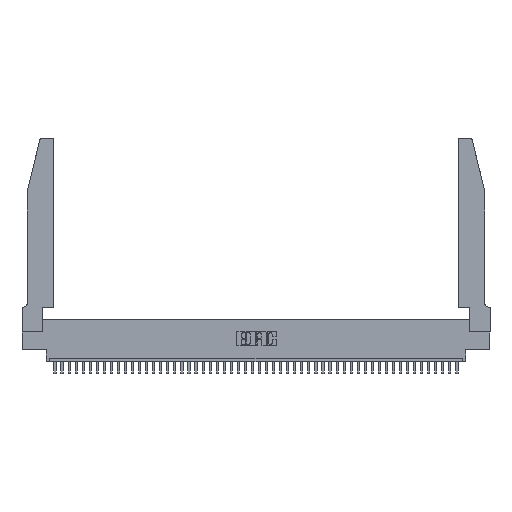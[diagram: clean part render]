
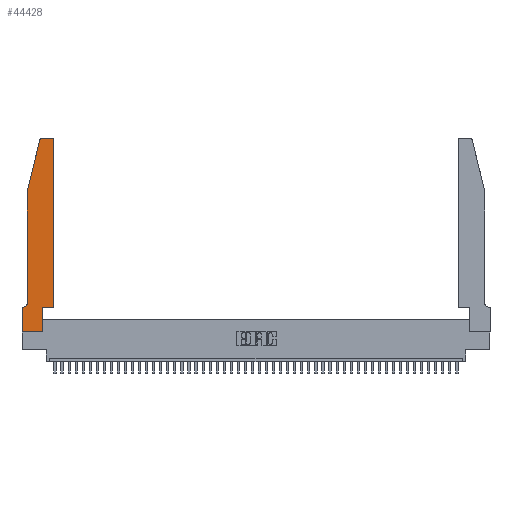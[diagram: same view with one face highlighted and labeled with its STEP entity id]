
A CAD part, top view. The second image highlights one B-rep face of the part: STEP entity #44428.
In plain terms, the highlighted planar face has unit normal (0, 0, 1).
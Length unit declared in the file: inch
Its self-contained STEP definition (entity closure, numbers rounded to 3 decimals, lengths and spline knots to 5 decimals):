
#929 = DIRECTION ( 'NONE',  ( -1., 0., 0. ) ) ;
#1763 = EDGE_CURVE ( 'NONE', #12668, #45169, #44004, .T. ) ;
#1873 = LINE ( 'NONE', #11984, #23789 ) ;
#2221 = EDGE_CURVE ( 'NONE', #45169, #33366, #1873, .T. ) ;
#2906 = EDGE_CURVE ( 'NONE', #33366, #6552, #17636, .T. ) ;
#4035 = ORIENTED_EDGE ( 'NONE', *, *, #28846, .T. ) ;
#4823 = VECTOR ( 'NONE', #13705, 39.37008 ) ;
#5790 = DIRECTION ( 'NONE',  ( 1., 0., 0. ) ) ;
#5920 = VERTEX_POINT ( 'NONE', #32987 ) ;
#6147 = EDGE_LOOP ( 'NONE', ( #6750, #25778, #36828, #45450, #25451, #10284, #23994, #35107, #44452, #25367, #8955, #4035 ) ) ;
#6552 = VERTEX_POINT ( 'NONE', #12943 ) ;
#6570 = EDGE_CURVE ( 'NONE', #5920, #10845, #46477, .T. ) ;
#6750 = ORIENTED_EDGE ( 'NONE', *, *, #9562, .T. ) ;
#7239 = CARTESIAN_POINT ( 'NONE',  ( 0.2865, 0.35, 0.37 ) ) ;
#8721 = LINE ( 'NONE', #35166, #18731 ) ;
#8955 = ORIENTED_EDGE ( 'NONE', *, *, #12081, .T. ) ;
#8992 = DIRECTION ( 'NONE',  ( -0.239, -0.971, 0. ) ) ;
#9445 = VERTEX_POINT ( 'NONE', #15338 ) ;
#9562 = EDGE_CURVE ( 'NONE', #10514, #5920, #22978, .T. ) ;
#10023 = EDGE_CURVE ( 'NONE', #6552, #16545, #29719, .T. ) ;
#10284 = ORIENTED_EDGE ( 'NONE', *, *, #2221, .T. ) ;
#10514 = VERTEX_POINT ( 'NONE', #44878 ) ;
#10845 = VERTEX_POINT ( 'NONE', #13922 ) ;
#11984 = CARTESIAN_POINT ( 'NONE',  ( 0.0755, 0.35, 0.37 ) ) ;
#12081 = EDGE_CURVE ( 'NONE', #36605, #31818, #8721, .T. ) ;
#12510 = FACE_OUTER_BOUND ( 'NONE', #6147, .T. ) ;
#12601 = VECTOR ( 'NONE', #39973, 39.37008 ) ;
#12668 = VERTEX_POINT ( 'NONE', #17203 ) ;
#12858 = PLANE ( 'NONE',  #36894 ) ;
#12943 = CARTESIAN_POINT ( 'NONE',  ( 0., 0., 0.37 ) ) ;
#13392 = CARTESIAN_POINT ( 'NONE',  ( 0.4505, 0.35, 0.37 ) ) ;
#13705 = DIRECTION ( 'NONE',  ( 1., 0., 0. ) ) ;
#13922 = CARTESIAN_POINT ( 'NONE',  ( 0.25487, 2.72718, 0.37 ) ) ;
#14198 = CARTESIAN_POINT ( 'NONE',  ( 0.0055, 0.35, 0.37 ) ) ;
#14454 = CARTESIAN_POINT ( 'NONE',  ( 0., 0.35, 0.37 ) ) ;
#15338 = CARTESIAN_POINT ( 'NONE',  ( 0.0755, 2., 0.37 ) ) ;
#15631 = VECTOR ( 'NONE', #17059, 39.37008 ) ;
#16433 = CARTESIAN_POINT ( 'NONE',  ( 0., 0.35, 0.37 ) ) ;
#16516 = CARTESIAN_POINT ( 'NONE',  ( 0.284, 2.72, 0.37 ) ) ;
#16545 = VERTEX_POINT ( 'NONE', #18893 ) ;
#17059 = DIRECTION ( 'NONE',  ( 1., 0., 0. ) ) ;
#17203 = CARTESIAN_POINT ( 'NONE',  ( 0.0755, 0.42, 0.37 ) ) ;
#17389 = DIRECTION ( 'NONE',  ( 0., 0., 1. ) ) ;
#17636 = LINE ( 'NONE', #18175, #12601 ) ;
#17657 = DIRECTION ( 'NONE',  ( 1., 0., 0. ) ) ;
#18054 = CARTESIAN_POINT ( 'NONE',  ( 0.4505, 2.72, 0.37 ) ) ;
#18175 = CARTESIAN_POINT ( 'NONE',  ( 0., 0., 0.37 ) ) ;
#18244 = DIRECTION ( 'NONE',  ( 0., 0., 1. ) ) ;
#18731 = VECTOR ( 'NONE', #32003, 39.37008 ) ;
#18893 = CARTESIAN_POINT ( 'NONE',  ( 0.2865, 0., 0.37 ) ) ;
#20066 = DIRECTION ( 'NONE',  ( 0., 0., 1. ) ) ;
#20583 = AXIS2_PLACEMENT_3D ( 'NONE', #28409, #17389, #35192 ) ;
#21056 = DIRECTION ( 'NONE',  ( 0., -1., 0. ) ) ;
#21186 = DIRECTION ( 'NONE',  ( 0., 0., -1. ) ) ;
#21301 = CARTESIAN_POINT ( 'NONE',  ( 0., 0., 0.37 ) ) ;
#22785 = LINE ( 'NONE', #13392, #4823 ) ;
#22978 = LINE ( 'NONE', #36343, #44322 ) ;
#23789 = VECTOR ( 'NONE', #929, 39.37008 ) ;
#23994 = ORIENTED_EDGE ( 'NONE', *, *, #2906, .T. ) ;
#25367 = ORIENTED_EDGE ( 'NONE', *, *, #41619, .T. ) ;
#25451 = ORIENTED_EDGE ( 'NONE', *, *, #1763, .T. ) ;
#25778 = ORIENTED_EDGE ( 'NONE', *, *, #6570, .T. ) ;
#27488 = CARTESIAN_POINT ( 'NONE',  ( 0.4505, 0.35, 0.37 ) ) ;
#28344 = VECTOR ( 'NONE', #42724, 39.37008 ) ;
#28409 = CARTESIAN_POINT ( 'NONE',  ( 0.4205, 2.72, 0.37 ) ) ;
#28846 = EDGE_CURVE ( 'NONE', #31818, #10514, #38286, .T. ) ;
#29719 = LINE ( 'NONE', #21301, #15631 ) ;
#31818 = VERTEX_POINT ( 'NONE', #18054 ) ;
#32003 = DIRECTION ( 'NONE',  ( 0., 1., 0. ) ) ;
#32987 = CARTESIAN_POINT ( 'NONE',  ( 0.284, 2.75, 0.37 ) ) ;
#33366 = VERTEX_POINT ( 'NONE', #14454 ) ;
#33807 = CARTESIAN_POINT ( 'NONE',  ( 0.0755, 2., 0.37 ) ) ;
#33955 = VECTOR ( 'NONE', #21056, 39.37008 ) ;
#34515 = AXIS2_PLACEMENT_3D ( 'NONE', #16516, #18244, #17657 ) ;
#35101 = CARTESIAN_POINT ( 'NONE',  ( 0.2865, 0.35, 0.37 ) ) ;
#35107 = ORIENTED_EDGE ( 'NONE', *, *, #10023, .T. ) ;
#35166 = CARTESIAN_POINT ( 'NONE',  ( 0.4505, 0.35, 0.37 ) ) ;
#35192 = DIRECTION ( 'NONE',  ( 1., 0., 0. ) ) ;
#35776 = DIRECTION ( 'NONE',  ( -1., 0., 0. ) ) ;
#36343 = CARTESIAN_POINT ( 'NONE',  ( 0.2605, 2.75, 0.37 ) ) ;
#36605 = VERTEX_POINT ( 'NONE', #27488 ) ;
#36828 = ORIENTED_EDGE ( 'NONE', *, *, #45481, .T. ) ;
#36894 = AXIS2_PLACEMENT_3D ( 'NONE', #16433, #20066, #5790 ) ;
#38286 = CIRCLE ( 'NONE', #20583, 0.03 ) ;
#39084 = CARTESIAN_POINT ( 'NONE',  ( 0.0055, 0.42, 0.37 ) ) ;
#39706 = AXIS2_PLACEMENT_3D ( 'NONE', #39084, #21186, #42379 ) ;
#39973 = DIRECTION ( 'NONE',  ( 0., -1., 0. ) ) ;
#40663 = VERTEX_POINT ( 'NONE', #7239 ) ;
#40673 = VECTOR ( 'NONE', #8992, 39.37008 ) ;
#41185 = LINE ( 'NONE', #46000, #33955 ) ;
#41619 = EDGE_CURVE ( 'NONE', #40663, #36605, #22785, .T. ) ;
#42379 = DIRECTION ( 'NONE',  ( -1., 0., 0. ) ) ;
#42724 = DIRECTION ( 'NONE',  ( 0., 1., 0. ) ) ;
#43895 = EDGE_CURVE ( 'NONE', #16545, #40663, #43957, .T. ) ;
#43957 = LINE ( 'NONE', #35101, #28344 ) ;
#44004 = CIRCLE ( 'NONE', #39706, 0.07 ) ;
#44322 = VECTOR ( 'NONE', #35776, 39.37008 ) ;
#44428 = ADVANCED_FACE ( 'NONE', ( #12510 ), #12858, .T. ) ;
#44452 = ORIENTED_EDGE ( 'NONE', *, *, #43895, .T. ) ;
#44878 = CARTESIAN_POINT ( 'NONE',  ( 0.4205, 2.75, 0.37 ) ) ;
#45169 = VERTEX_POINT ( 'NONE', #14198 ) ;
#45450 = ORIENTED_EDGE ( 'NONE', *, *, #45754, .T. ) ;
#45481 = EDGE_CURVE ( 'NONE', #10845, #9445, #45767, .T. ) ;
#45754 = EDGE_CURVE ( 'NONE', #9445, #12668, #41185, .T. ) ;
#45767 = LINE ( 'NONE', #33807, #40673 ) ;
#46000 = CARTESIAN_POINT ( 'NONE',  ( 0.0755, 2., 0.37 ) ) ;
#46477 = CIRCLE ( 'NONE', #34515, 0.03 ) ;
